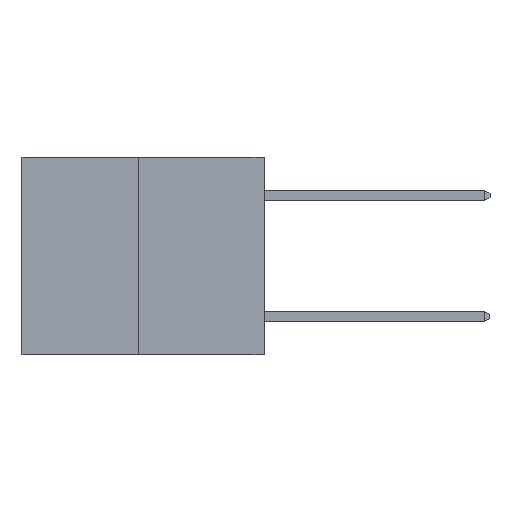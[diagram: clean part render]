
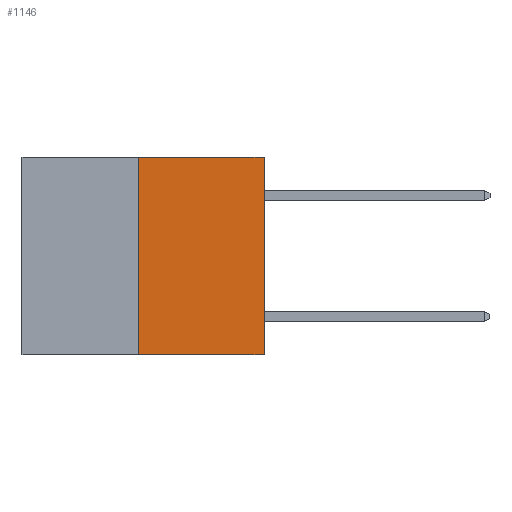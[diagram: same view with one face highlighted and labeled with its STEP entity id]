
A CAD part, left-side view. The second image highlights one B-rep face of the part: STEP entity #1146.
In plain terms, the highlighted planar face has unit normal (-1, 0, 0).
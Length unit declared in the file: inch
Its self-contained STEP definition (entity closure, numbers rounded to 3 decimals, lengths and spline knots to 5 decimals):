
#718 = CARTESIAN_POINT ( 'NONE',  ( 0., 0., -0.49 ) ) ;
#1146 = ADVANCED_FACE ( 'NONE', ( #15849 ), #9591, .F. ) ;
#1208 = LINE ( 'NONE', #2645, #10761 ) ;
#1847 = CARTESIAN_POINT ( 'NONE',  ( 0., 0., 0. ) ) ;
#2086 = LINE ( 'NONE', #5056, #7291 ) ;
#2645 = CARTESIAN_POINT ( 'NONE',  ( 0., 0.312, -0.49 ) ) ;
#3581 = ORIENTED_EDGE ( 'NONE', *, *, #14939, .F. ) ;
#4289 = DIRECTION ( 'NONE',  ( 0., -1., 0. ) ) ;
#4579 = CARTESIAN_POINT ( 'NONE',  ( 0., 0.312, 0. ) ) ;
#5056 = CARTESIAN_POINT ( 'NONE',  ( 0., 0.6, 0. ) ) ;
#5244 = VERTEX_POINT ( 'NONE', #12193 ) ;
#5616 = ORIENTED_EDGE ( 'NONE', *, *, #12729, .T. ) ;
#5835 = VERTEX_POINT ( 'NONE', #10625 ) ;
#6530 = DIRECTION ( 'NONE',  ( 0., 0., 1. ) ) ;
#6584 = VERTEX_POINT ( 'NONE', #718 ) ;
#6759 = DIRECTION ( 'NONE',  ( 0., 0., -1. ) ) ;
#7291 = VECTOR ( 'NONE', #12386, 39.37008 ) ;
#7875 = LINE ( 'NONE', #1847, #16335 ) ;
#8024 = DIRECTION ( 'NONE',  ( 1., 0., 0. ) ) ;
#9591 = PLANE ( 'NONE',  #13603 ) ;
#9857 = EDGE_CURVE ( 'NONE', #6584, #5835, #7875, .T. ) ;
#10544 = EDGE_LOOP ( 'NONE', ( #14563, #5616, #17374, #3581 ) ) ;
#10555 = DIRECTION ( 'NONE',  ( 0., 0., 1. ) ) ;
#10625 = CARTESIAN_POINT ( 'NONE',  ( 0., 0., 0. ) ) ;
#10761 = VECTOR ( 'NONE', #6530, 39.37008 ) ;
#11400 = VERTEX_POINT ( 'NONE', #4579 ) ;
#12193 = CARTESIAN_POINT ( 'NONE',  ( 0., 0.312, -0.49 ) ) ;
#12386 = DIRECTION ( 'NONE',  ( 0., -1., 0. ) ) ;
#12587 = CARTESIAN_POINT ( 'NONE',  ( 0., 0.6, -0.49 ) ) ;
#12729 = EDGE_CURVE ( 'NONE', #5244, #6584, #16445, .T. ) ;
#13603 = AXIS2_PLACEMENT_3D ( 'NONE', #15132, #8024, #6759 ) ;
#14288 = EDGE_CURVE ( 'NONE', #5244, #11400, #1208, .T. ) ;
#14563 = ORIENTED_EDGE ( 'NONE', *, *, #14288, .F. ) ;
#14939 = EDGE_CURVE ( 'NONE', #11400, #5835, #2086, .T. ) ;
#15132 = CARTESIAN_POINT ( 'NONE',  ( 0., 0.6, 0. ) ) ;
#15849 = FACE_OUTER_BOUND ( 'NONE', #10544, .T. ) ;
#16335 = VECTOR ( 'NONE', #10555, 39.37008 ) ;
#16445 = LINE ( 'NONE', #12587, #17550 ) ;
#17374 = ORIENTED_EDGE ( 'NONE', *, *, #9857, .T. ) ;
#17550 = VECTOR ( 'NONE', #4289, 39.37008 ) ;
